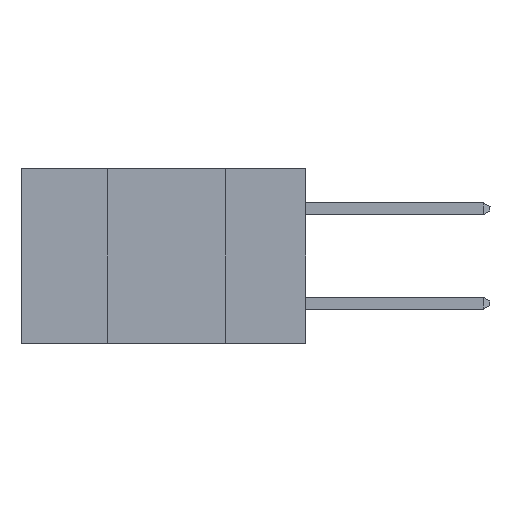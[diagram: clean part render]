
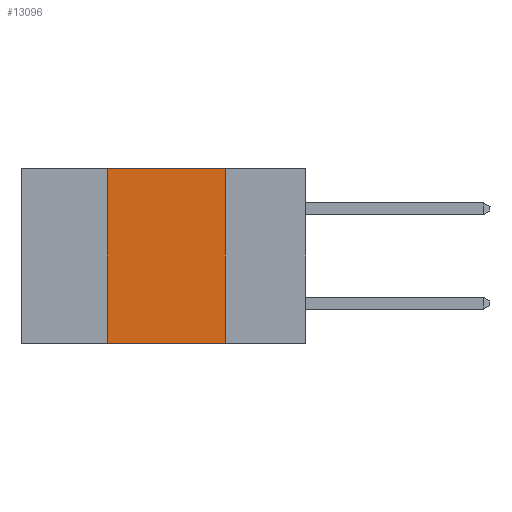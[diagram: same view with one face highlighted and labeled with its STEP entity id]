
A CAD part, left-side view. The second image highlights one B-rep face of the part: STEP entity #13096.
In plain terms, the highlighted planar face has unit normal (-1, 0, 0).
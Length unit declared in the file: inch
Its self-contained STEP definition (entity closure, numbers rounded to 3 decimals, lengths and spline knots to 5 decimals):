
#1050 = EDGE_LOOP ( 'NONE', ( #16082, #9050, #11101, #16749 ) ) ;
#1193 = VERTEX_POINT ( 'NONE', #13097 ) ;
#1304 = VERTEX_POINT ( 'NONE', #6449 ) ;
#4345 = DIRECTION ( 'NONE',  ( 1., 0., 0. ) ) ;
#4730 = CARTESIAN_POINT ( 'NONE',  ( 0., 0.42, -0.37 ) ) ;
#5371 = EDGE_CURVE ( 'NONE', #20785, #1304, #7154, .T. ) ;
#6449 = CARTESIAN_POINT ( 'NONE',  ( 0., 0.17, -0.37 ) ) ;
#7154 = LINE ( 'NONE', #24449, #19036 ) ;
#9050 = ORIENTED_EDGE ( 'NONE', *, *, #23765, .F. ) ;
#9487 = CARTESIAN_POINT ( 'NONE',  ( 0., 0.6, 0. ) ) ;
#10342 = VERTEX_POINT ( 'NONE', #4730 ) ;
#11101 = ORIENTED_EDGE ( 'NONE', *, *, #23416, .F. ) ;
#12295 = DIRECTION ( 'NONE',  ( 0., 0., 1. ) ) ;
#12342 = VECTOR ( 'NONE', #12295, 39.37008 ) ;
#13096 = ADVANCED_FACE ( 'NONE', ( #29563 ), #28356, .F. ) ;
#13097 = CARTESIAN_POINT ( 'NONE',  ( 0., 0.42, 0. ) ) ;
#14113 = DIRECTION ( 'NONE',  ( 0., -1., 0. ) ) ;
#14491 = CARTESIAN_POINT ( 'NONE',  ( 0., 0.6, -0.37 ) ) ;
#14619 = LINE ( 'NONE', #14491, #25460 ) ;
#14965 = CARTESIAN_POINT ( 'NONE',  ( 0., 0.42, 0. ) ) ;
#15604 = AXIS2_PLACEMENT_3D ( 'NONE', #9487, #4345, #16674 ) ;
#15671 = LINE ( 'NONE', #14965, #12342 ) ;
#16007 = LINE ( 'NONE', #19539, #27971 ) ;
#16082 = ORIENTED_EDGE ( 'NONE', *, *, #5371, .F. ) ;
#16674 = DIRECTION ( 'NONE',  ( 0., 0., -1. ) ) ;
#16749 = ORIENTED_EDGE ( 'NONE', *, *, #22632, .T. ) ;
#19036 = VECTOR ( 'NONE', #20082, 39.37008 ) ;
#19539 = CARTESIAN_POINT ( 'NONE',  ( 0., 0.6, 0. ) ) ;
#20082 = DIRECTION ( 'NONE',  ( 0., 0., -1. ) ) ;
#20785 = VERTEX_POINT ( 'NONE', #21889 ) ;
#21370 = DIRECTION ( 'NONE',  ( 0., -1., 0. ) ) ;
#21889 = CARTESIAN_POINT ( 'NONE',  ( 0., 0.17, 0. ) ) ;
#22632 = EDGE_CURVE ( 'NONE', #10342, #1304, #14619, .T. ) ;
#23416 = EDGE_CURVE ( 'NONE', #10342, #1193, #15671, .T. ) ;
#23765 = EDGE_CURVE ( 'NONE', #1193, #20785, #16007, .T. ) ;
#24449 = CARTESIAN_POINT ( 'NONE',  ( 0., 0.17, 0. ) ) ;
#25460 = VECTOR ( 'NONE', #21370, 39.37008 ) ;
#27971 = VECTOR ( 'NONE', #14113, 39.37008 ) ;
#28356 = PLANE ( 'NONE',  #15604 ) ;
#29563 = FACE_OUTER_BOUND ( 'NONE', #1050, .T. ) ;
